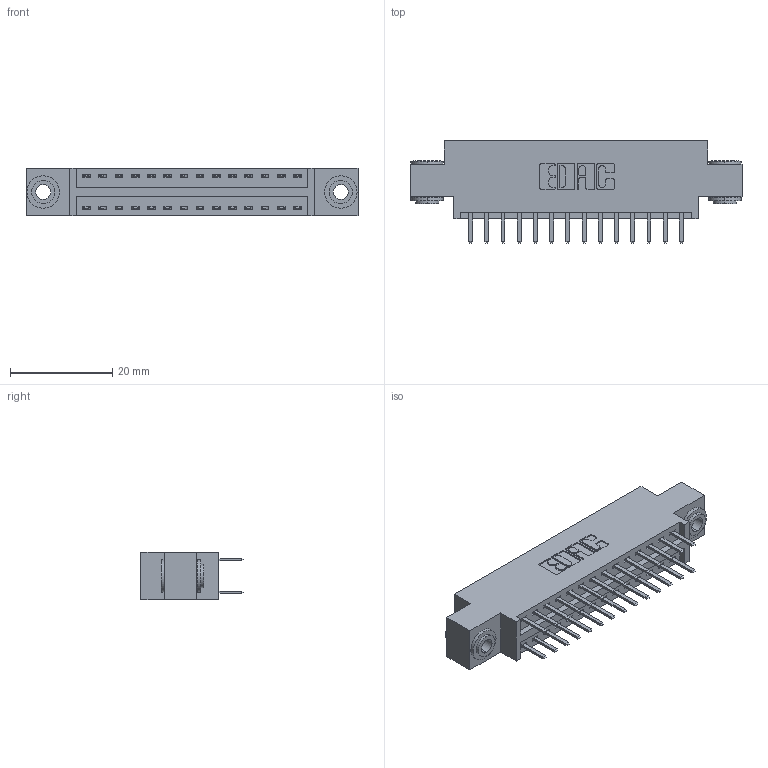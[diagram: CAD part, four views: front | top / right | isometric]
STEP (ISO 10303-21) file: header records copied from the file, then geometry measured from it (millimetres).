
FILE_DESCRIPTION (( 'STEP AP203' ), '1' );
FILE_NAME ('346-028-520-803.STEP', '2022-05-19T03:38:14', ( '' ), ( '' ), 'SwSTEP 2.0', 'SolidWorks 2020', '' );
FILE_SCHEMA (( 'CONFIG_CONTROL_DESIGN' ));
Length unit declared in the file: inch
Products named in the file (4): 345-292-001_345-293-120; 346-028-520-803; 346 Part_0.170 Offset - 0.156 Dia-TH; 345-250-002_345-250-002-102
Assembly tree (31 placements, depth 2):
  346-028-520-803
    346 Part_0.170 Offset - 0.156 Dia-TH
    345-292-001_345-293-120  x28
    345-250-002_345-250-002-102  x2
Bounding box: 65.02 x 20.02 x 9.4 mm (x, y, z)
Volume: 5957.6 mm3; surface area: 8148.5 mm2
Topology: 31 solids, 31 shells, 1746 faces, 5017 edges, 3266 vertices
Faces by surface type: plane 1140, cylinder 598, cone 8
Entity records: 14218 total; most frequent: CARTESIAN_POINT 2377, ORIENTED_EDGE 2290, DIRECTION 2163, EDGE_CURVE 1145, VECTOR 929, LINE 929, VERTEX_POINT 758, AXIS2_PLACEMENT_3D 617
